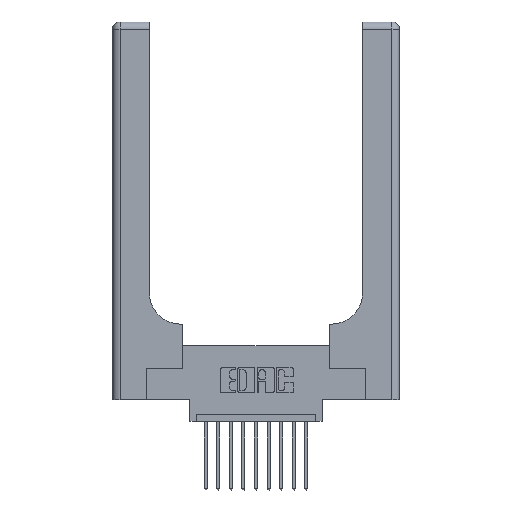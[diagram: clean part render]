
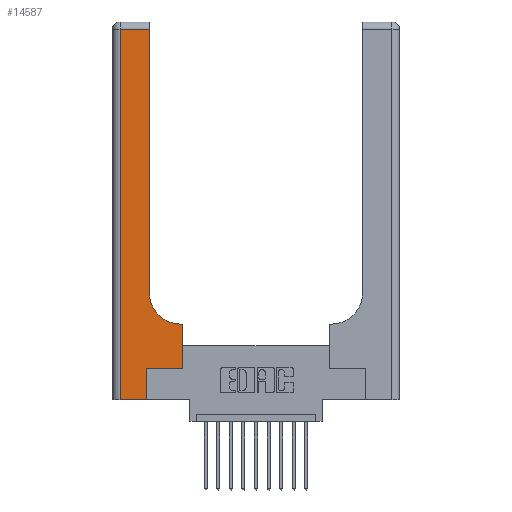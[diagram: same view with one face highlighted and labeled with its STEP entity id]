
A CAD part, top view. The second image highlights one B-rep face of the part: STEP entity #14587.
In plain terms, the highlighted planar face has unit normal (0, 0, 1).
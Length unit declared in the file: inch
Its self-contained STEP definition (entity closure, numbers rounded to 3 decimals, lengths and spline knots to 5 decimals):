
#231 = ORIENTED_EDGE ( 'NONE', *, *, #2398, .T. ) ;
#344 = LINE ( 'NONE', #2961, #14170 ) ;
#696 = ORIENTED_EDGE ( 'NONE', *, *, #10638, .T. ) ;
#723 = VERTEX_POINT ( 'NONE', #13948 ) ;
#815 = FACE_OUTER_BOUND ( 'NONE', #15235, .T. ) ;
#993 = CARTESIAN_POINT ( 'NONE',  ( 0., 3., 0.37 ) ) ;
#1073 = EDGE_CURVE ( 'NONE', #1231, #13592, #1892, .T. ) ;
#1231 = VERTEX_POINT ( 'NONE', #10795 ) ;
#1338 = AXIS2_PLACEMENT_3D ( 'NONE', #993, #13871, #3505 ) ;
#1339 = LINE ( 'NONE', #2661, #15525 ) ;
#1464 = ORIENTED_EDGE ( 'NONE', *, *, #4070, .T. ) ;
#1691 = DIRECTION ( 'NONE',  ( 0., 0., -1. ) ) ;
#1892 = LINE ( 'NONE', #16185, #8487 ) ;
#1949 = DIRECTION ( 'NONE',  ( 0., 1., 0. ) ) ;
#2014 = LINE ( 'NONE', #9746, #7789 ) ;
#2146 = LINE ( 'NONE', #13806, #15344 ) ;
#2237 = PLANE ( 'NONE',  #1338 ) ;
#2398 = EDGE_CURVE ( 'NONE', #7254, #3362, #6255, .T. ) ;
#2661 = CARTESIAN_POINT ( 'NONE',  ( 0., 0., 0.37 ) ) ;
#2961 = CARTESIAN_POINT ( 'NONE',  ( 0., 2.94, 0.37 ) ) ;
#3362 = VERTEX_POINT ( 'NONE', #5364 ) ;
#3505 = DIRECTION ( 'NONE',  ( -1., 0., 0. ) ) ;
#3990 = CARTESIAN_POINT ( 'NONE',  ( 0.5585, 0.6, 0.37 ) ) ;
#4070 = EDGE_CURVE ( 'NONE', #723, #1231, #2014, .T. ) ;
#4729 = EDGE_CURVE ( 'NONE', #9628, #8043, #5772, .T. ) ;
#4783 = DIRECTION ( 'NONE',  ( 0., -1., 0. ) ) ;
#5156 = EDGE_CURVE ( 'NONE', #13475, #723, #14193, .T. ) ;
#5364 = CARTESIAN_POINT ( 'NONE',  ( 0.06, 0., 0.37 ) ) ;
#5573 = EDGE_CURVE ( 'NONE', #8308, #7254, #344, .T. ) ;
#5772 = CIRCLE ( 'NONE', #6635, 0.25 ) ;
#5979 = EDGE_CURVE ( 'NONE', #8043, #8308, #2146, .T. ) ;
#6099 = EDGE_CURVE ( 'NONE', #3362, #13475, #1339, .T. ) ;
#6154 = CARTESIAN_POINT ( 'NONE',  ( 0.2915, 2.94, 0.37 ) ) ;
#6255 = LINE ( 'NONE', #9797, #16440 ) ;
#6367 = VECTOR ( 'NONE', #6876, 39.37008 ) ;
#6635 = AXIS2_PLACEMENT_3D ( 'NONE', #14568, #1691, #11986 ) ;
#6876 = DIRECTION ( 'NONE',  ( 0., 1., 0. ) ) ;
#7064 = CARTESIAN_POINT ( 'NONE',  ( 0.2915, 0.85, 0.37 ) ) ;
#7254 = VERTEX_POINT ( 'NONE', #11392 ) ;
#7662 = DIRECTION ( 'NONE',  ( -1., 0., 0. ) ) ;
#7789 = VECTOR ( 'NONE', #16013, 39.37008 ) ;
#8043 = VERTEX_POINT ( 'NONE', #7064 ) ;
#8237 = ORIENTED_EDGE ( 'NONE', *, *, #6099, .T. ) ;
#8280 = ORIENTED_EDGE ( 'NONE', *, *, #5156, .T. ) ;
#8308 = VERTEX_POINT ( 'NONE', #6154 ) ;
#8487 = VECTOR ( 'NONE', #1949, 39.37008 ) ;
#9141 = ORIENTED_EDGE ( 'NONE', *, *, #1073, .T. ) ;
#9628 = VERTEX_POINT ( 'NONE', #16387 ) ;
#9746 = CARTESIAN_POINT ( 'NONE',  ( 0.269, 0.25, 0.37 ) ) ;
#9797 = CARTESIAN_POINT ( 'NONE',  ( 0.06, 3., 0.37 ) ) ;
#10497 = VECTOR ( 'NONE', #7662, 39.37008 ) ;
#10638 = EDGE_CURVE ( 'NONE', #13592, #9628, #16497, .T. ) ;
#10795 = CARTESIAN_POINT ( 'NONE',  ( 0.5585, 0.25, 0.37 ) ) ;
#10893 = ORIENTED_EDGE ( 'NONE', *, *, #5573, .T. ) ;
#11392 = CARTESIAN_POINT ( 'NONE',  ( 0.06, 2.94, 0.37 ) ) ;
#11986 = DIRECTION ( 'NONE',  ( 1., 0., 0. ) ) ;
#12910 = ORIENTED_EDGE ( 'NONE', *, *, #5979, .T. ) ;
#13475 = VERTEX_POINT ( 'NONE', #15550 ) ;
#13592 = VERTEX_POINT ( 'NONE', #3990 ) ;
#13806 = CARTESIAN_POINT ( 'NONE',  ( 0.2915, 3., 0.37 ) ) ;
#13871 = DIRECTION ( 'NONE',  ( 0., 0., -1. ) ) ;
#13948 = CARTESIAN_POINT ( 'NONE',  ( 0.269, 0.25, 0.37 ) ) ;
#14134 = DIRECTION ( 'NONE',  ( 1., 0., 0. ) ) ;
#14170 = VECTOR ( 'NONE', #15742, 39.37008 ) ;
#14193 = LINE ( 'NONE', #15762, #6367 ) ;
#14228 = CARTESIAN_POINT ( 'NONE',  ( 0.2915, 0.6, 0.37 ) ) ;
#14568 = CARTESIAN_POINT ( 'NONE',  ( 0.5415, 0.85, 0.37 ) ) ;
#14587 = ADVANCED_FACE ( 'NONE', ( #815 ), #2237, .F. ) ;
#15232 = DIRECTION ( 'NONE',  ( 0., 1., 0. ) ) ;
#15235 = EDGE_LOOP ( 'NONE', ( #12910, #10893, #231, #8237, #8280, #1464, #9141, #696, #15327 ) ) ;
#15327 = ORIENTED_EDGE ( 'NONE', *, *, #4729, .T. ) ;
#15344 = VECTOR ( 'NONE', #15232, 39.37008 ) ;
#15525 = VECTOR ( 'NONE', #14134, 39.37008 ) ;
#15550 = CARTESIAN_POINT ( 'NONE',  ( 0.269, 0., 0.37 ) ) ;
#15742 = DIRECTION ( 'NONE',  ( -1., 0., 0. ) ) ;
#15762 = CARTESIAN_POINT ( 'NONE',  ( 0.269, 0., 0.37 ) ) ;
#16013 = DIRECTION ( 'NONE',  ( 1., 0., 0. ) ) ;
#16185 = CARTESIAN_POINT ( 'NONE',  ( 0.5585, 0.25, 0.37 ) ) ;
#16387 = CARTESIAN_POINT ( 'NONE',  ( 0.5415, 0.6, 0.37 ) ) ;
#16440 = VECTOR ( 'NONE', #4783, 39.37008 ) ;
#16497 = LINE ( 'NONE', #14228, #10497 ) ;
